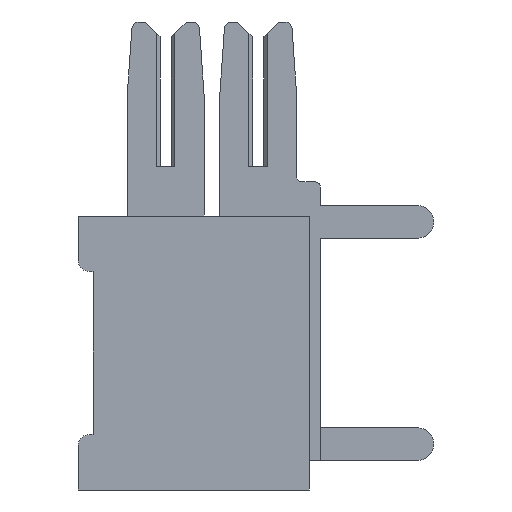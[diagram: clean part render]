
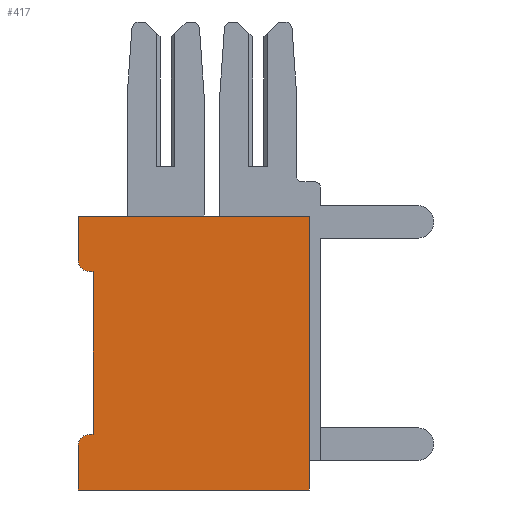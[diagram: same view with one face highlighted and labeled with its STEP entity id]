
A CAD part, left-side view. The second image highlights one B-rep face of the part: STEP entity #417.
In plain terms, the highlighted planar face has unit normal (-1, 0, 0).
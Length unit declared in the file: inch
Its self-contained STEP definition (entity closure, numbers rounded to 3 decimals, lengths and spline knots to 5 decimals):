
#21 = CIRCLE ( 'NONE', #5799, 0.015 ) ;
#417 = ADVANCED_FACE ( 'NONE', ( #4275 ), #598, .T. ) ;
#598 = PLANE ( 'NONE',  #1215 ) ;
#637 = DIRECTION ( 'NONE',  ( -1., 0., 0. ) ) ;
#696 = VECTOR ( 'NONE', #6852, 39.37008 ) ;
#986 = ORIENTED_EDGE ( 'NONE', *, *, #2379, .F. ) ;
#1215 = AXIS2_PLACEMENT_3D ( 'NONE', #10621, #11535, #11499 ) ;
#1250 = EDGE_CURVE ( 'NONE', #5819, #7786, #21, .T. ) ;
#1328 = EDGE_CURVE ( 'NONE', #10307, #7363, #5015, .T. ) ;
#1573 = CARTESIAN_POINT ( 'NONE',  ( 0., 0., -0.37 ) ) ;
#1777 = EDGE_CURVE ( 'NONE', #10307, #7786, #4583, .T. ) ;
#1842 = LINE ( 'NONE', #8902, #10996 ) ;
#1935 = CARTESIAN_POINT ( 'NONE',  ( 0., 0.312, -0.06 ) ) ;
#1992 = DIRECTION ( 'NONE',  ( 0., 0., 1. ) ) ;
#2123 = CARTESIAN_POINT ( 'NONE',  ( 0., 0.312, -0.37 ) ) ;
#2197 = CARTESIAN_POINT ( 'NONE',  ( 0., 0.292, -0.075 ) ) ;
#2207 = DIRECTION ( 'NONE',  ( 0., 0., 1. ) ) ;
#2379 = EDGE_CURVE ( 'NONE', #5819, #11180, #1842, .T. ) ;
#2453 = CIRCLE ( 'NONE', #3160, 0.015 ) ;
#2572 = LINE ( 'NONE', #6054, #6000 ) ;
#2716 = DIRECTION ( 'NONE',  ( 0., -1., 0. ) ) ;
#2775 = VERTEX_POINT ( 'NONE', #5225 ) ;
#2995 = LINE ( 'NONE', #8444, #8531 ) ;
#3160 = AXIS2_PLACEMENT_3D ( 'NONE', #5281, #637, #6118 ) ;
#3172 = ORIENTED_EDGE ( 'NONE', *, *, #4398, .T. ) ;
#3247 = EDGE_CURVE ( 'NONE', #11180, #10686, #2995, .T. ) ;
#3667 = ORIENTED_EDGE ( 'NONE', *, *, #3247, .F. ) ;
#3819 = CARTESIAN_POINT ( 'NONE',  ( 0., 0., 0. ) ) ;
#4058 = CARTESIAN_POINT ( 'NONE',  ( 0., 0., 0. ) ) ;
#4245 = DIRECTION ( 'NONE',  ( 0., -1., 0. ) ) ;
#4275 = FACE_OUTER_BOUND ( 'NONE', #10399, .T. ) ;
#4356 = CARTESIAN_POINT ( 'NONE',  ( 0., 0.292, -0.295 ) ) ;
#4398 = EDGE_CURVE ( 'NONE', #7363, #6641, #2572, .T. ) ;
#4583 = LINE ( 'NONE', #5222, #11581 ) ;
#5015 = LINE ( 'NONE', #1573, #6594 ) ;
#5222 = CARTESIAN_POINT ( 'NONE',  ( 0., 0.312, -0.37 ) ) ;
#5225 = CARTESIAN_POINT ( 'NONE',  ( 0., 0.297, -0.075 ) ) ;
#5263 = DIRECTION ( 'NONE',  ( 0., -1., 0. ) ) ;
#5281 = CARTESIAN_POINT ( 'NONE',  ( 0., 0.297, -0.06 ) ) ;
#5329 = ORIENTED_EDGE ( 'NONE', *, *, #1777, .F. ) ;
#5408 = EDGE_CURVE ( 'NONE', #10686, #2775, #5839, .T. ) ;
#5470 = CARTESIAN_POINT ( 'NONE',  ( 0., 0.297, -0.295 ) ) ;
#5798 = VERTEX_POINT ( 'NONE', #1935 ) ;
#5799 = AXIS2_PLACEMENT_3D ( 'NONE', #11023, #9122, #7352 ) ;
#5819 = VERTEX_POINT ( 'NONE', #5470 ) ;
#5839 = LINE ( 'NONE', #6733, #696 ) ;
#5872 = VERTEX_POINT ( 'NONE', #11011 ) ;
#6000 = VECTOR ( 'NONE', #11556, 39.37008 ) ;
#6054 = CARTESIAN_POINT ( 'NONE',  ( 0., 0., -0.37 ) ) ;
#6107 = ORIENTED_EDGE ( 'NONE', *, *, #9268, .T. ) ;
#6118 = DIRECTION ( 'NONE',  ( 0., 0., 1. ) ) ;
#6214 = ORIENTED_EDGE ( 'NONE', *, *, #5408, .F. ) ;
#6594 = VECTOR ( 'NONE', #4245, 39.37008 ) ;
#6641 = VERTEX_POINT ( 'NONE', #4058 ) ;
#6733 = CARTESIAN_POINT ( 'NONE',  ( 0., 0.312, -0.075 ) ) ;
#6852 = DIRECTION ( 'NONE',  ( 0., 1., 0. ) ) ;
#6969 = ORIENTED_EDGE ( 'NONE', *, *, #1328, .T. ) ;
#7352 = DIRECTION ( 'NONE',  ( 0., 0., 1. ) ) ;
#7363 = VERTEX_POINT ( 'NONE', #9420 ) ;
#7444 = ORIENTED_EDGE ( 'NONE', *, *, #10122, .F. ) ;
#7786 = VERTEX_POINT ( 'NONE', #11197 ) ;
#8295 = LINE ( 'NONE', #3819, #8418 ) ;
#8418 = VECTOR ( 'NONE', #2716, 39.37008 ) ;
#8444 = CARTESIAN_POINT ( 'NONE',  ( 0., 0.292, -0.295 ) ) ;
#8531 = VECTOR ( 'NONE', #1992, 39.37008 ) ;
#8619 = CARTESIAN_POINT ( 'NONE',  ( 0., 0.312, -0.37 ) ) ;
#8685 = VECTOR ( 'NONE', #2207, 39.37008 ) ;
#8902 = CARTESIAN_POINT ( 'NONE',  ( 0., 0.312, -0.295 ) ) ;
#8956 = ORIENTED_EDGE ( 'NONE', *, *, #9745, .F. ) ;
#8985 = LINE ( 'NONE', #2123, #8685 ) ;
#9122 = DIRECTION ( 'NONE',  ( -1., 0., 0. ) ) ;
#9268 = EDGE_CURVE ( 'NONE', #5798, #2775, #2453, .T. ) ;
#9420 = CARTESIAN_POINT ( 'NONE',  ( 0., 0., -0.37 ) ) ;
#9675 = DIRECTION ( 'NONE',  ( 0., 0., 1. ) ) ;
#9745 = EDGE_CURVE ( 'NONE', #5872, #6641, #8295, .T. ) ;
#10122 = EDGE_CURVE ( 'NONE', #5798, #5872, #8985, .T. ) ;
#10307 = VERTEX_POINT ( 'NONE', #8619 ) ;
#10399 = EDGE_LOOP ( 'NONE', ( #7444, #6107, #6214, #3667, #986, #11686, #5329, #6969, #3172, #8956 ) ) ;
#10621 = CARTESIAN_POINT ( 'NONE',  ( 0., 0., -0.37 ) ) ;
#10686 = VERTEX_POINT ( 'NONE', #2197 ) ;
#10996 = VECTOR ( 'NONE', #5263, 39.37008 ) ;
#11011 = CARTESIAN_POINT ( 'NONE',  ( 0., 0.312, 0. ) ) ;
#11023 = CARTESIAN_POINT ( 'NONE',  ( 0., 0.297, -0.31 ) ) ;
#11180 = VERTEX_POINT ( 'NONE', #4356 ) ;
#11197 = CARTESIAN_POINT ( 'NONE',  ( 0., 0.312, -0.31 ) ) ;
#11499 = DIRECTION ( 'NONE',  ( 0., 0., 1. ) ) ;
#11535 = DIRECTION ( 'NONE',  ( -1., 0., 0. ) ) ;
#11556 = DIRECTION ( 'NONE',  ( 0., 0., 1. ) ) ;
#11581 = VECTOR ( 'NONE', #9675, 39.37008 ) ;
#11686 = ORIENTED_EDGE ( 'NONE', *, *, #1250, .T. ) ;
